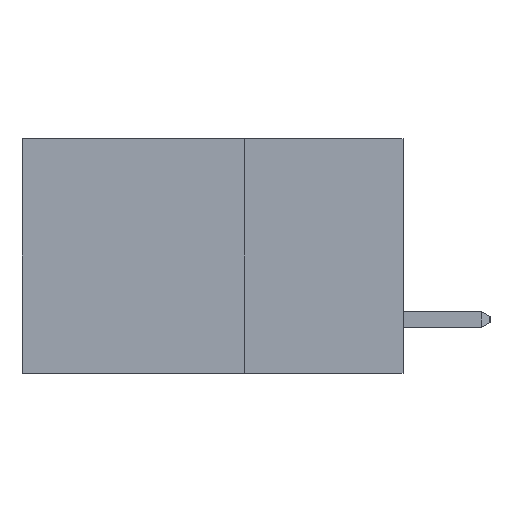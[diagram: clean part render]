
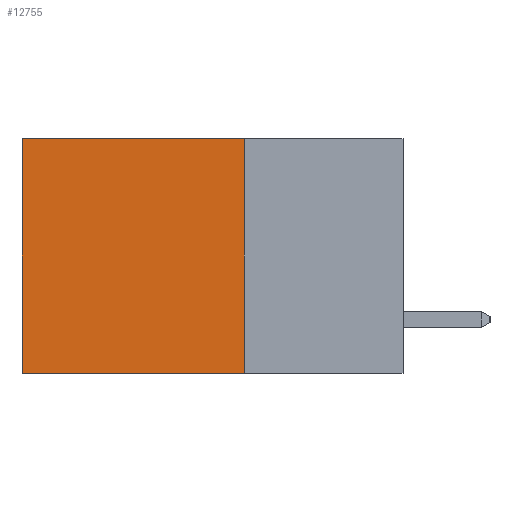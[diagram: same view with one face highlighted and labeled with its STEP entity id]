
A CAD part, left-side view. The second image highlights one B-rep face of the part: STEP entity #12755.
In plain terms, the highlighted planar face has unit normal (-1, 0, 0).
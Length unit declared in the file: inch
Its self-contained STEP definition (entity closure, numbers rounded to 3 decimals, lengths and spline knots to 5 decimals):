
#578 = CARTESIAN_POINT ( 'NONE',  ( 0.2875, 0.6, 0. ) ) ;
#801 = DIRECTION ( 'NONE',  ( 1., 0., 0. ) ) ;
#1498 = LINE ( 'NONE', #6249, #9243 ) ;
#1895 = FACE_OUTER_BOUND ( 'NONE', #9462, .T. ) ;
#2256 = CARTESIAN_POINT ( 'NONE',  ( 0.2875, 0.25, -0.37 ) ) ;
#2930 = CARTESIAN_POINT ( 'NONE',  ( 0.2875, 0.25, 0. ) ) ;
#3211 = VERTEX_POINT ( 'NONE', #9681 ) ;
#3294 = DIRECTION ( 'NONE',  ( 0., 1., 0. ) ) ;
#3379 = ORIENTED_EDGE ( 'NONE', *, *, #7632, .F. ) ;
#3640 = VERTEX_POINT ( 'NONE', #8826 ) ;
#3750 = EDGE_CURVE ( 'NONE', #4618, #7221, #4779, .T. ) ;
#3835 = VECTOR ( 'NONE', #3294, 39.37008 ) ;
#4269 = ORIENTED_EDGE ( 'NONE', *, *, #3750, .T. ) ;
#4618 = VERTEX_POINT ( 'NONE', #5121 ) ;
#4695 = DIRECTION ( 'NONE',  ( 0., 0., -1. ) ) ;
#4779 = LINE ( 'NONE', #8760, #9359 ) ;
#5121 = CARTESIAN_POINT ( 'NONE',  ( 0.2875, 0.25, 0. ) ) ;
#6108 = VECTOR ( 'NONE', #12083, 39.37008 ) ;
#6249 = CARTESIAN_POINT ( 'NONE',  ( 0.2875, 0.25, 0. ) ) ;
#6671 = EDGE_CURVE ( 'NONE', #7221, #3211, #10248, .T. ) ;
#7219 = EDGE_CURVE ( 'NONE', #4618, #3640, #1498, .T. ) ;
#7221 = VERTEX_POINT ( 'NONE', #578 ) ;
#7632 = EDGE_CURVE ( 'NONE', #3640, #3211, #8257, .T. ) ;
#7703 = PLANE ( 'NONE',  #7877 ) ;
#7877 = AXIS2_PLACEMENT_3D ( 'NONE', #2930, #801, #4695 ) ;
#8257 = LINE ( 'NONE', #2256, #3835 ) ;
#8760 = CARTESIAN_POINT ( 'NONE',  ( 0.2875, 0.25, 0. ) ) ;
#8826 = CARTESIAN_POINT ( 'NONE',  ( 0.2875, 0.25, -0.37 ) ) ;
#9204 = CARTESIAN_POINT ( 'NONE',  ( 0.2875, 0.6, 0. ) ) ;
#9243 = VECTOR ( 'NONE', #12387, 39.37008 ) ;
#9359 = VECTOR ( 'NONE', #12748, 39.37008 ) ;
#9462 = EDGE_LOOP ( 'NONE', ( #9506, #3379, #11089, #4269 ) ) ;
#9506 = ORIENTED_EDGE ( 'NONE', *, *, #6671, .T. ) ;
#9681 = CARTESIAN_POINT ( 'NONE',  ( 0.2875, 0.6, -0.37 ) ) ;
#10248 = LINE ( 'NONE', #9204, #6108 ) ;
#11089 = ORIENTED_EDGE ( 'NONE', *, *, #7219, .F. ) ;
#12083 = DIRECTION ( 'NONE',  ( 0., 0., -1. ) ) ;
#12387 = DIRECTION ( 'NONE',  ( 0., 0., -1. ) ) ;
#12748 = DIRECTION ( 'NONE',  ( 0., 1., 0. ) ) ;
#12755 = ADVANCED_FACE ( 'NONE', ( #1895 ), #7703, .F. ) ;
